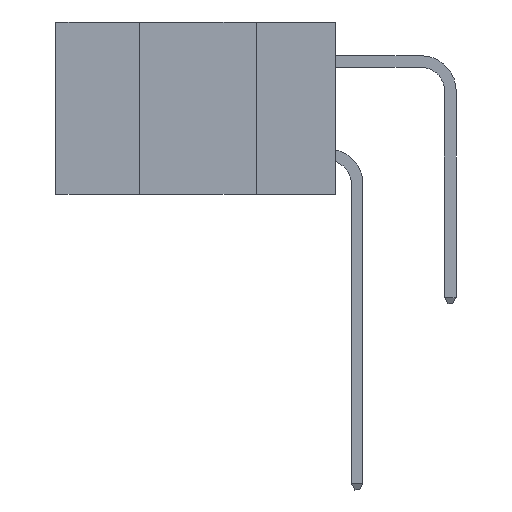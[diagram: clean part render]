
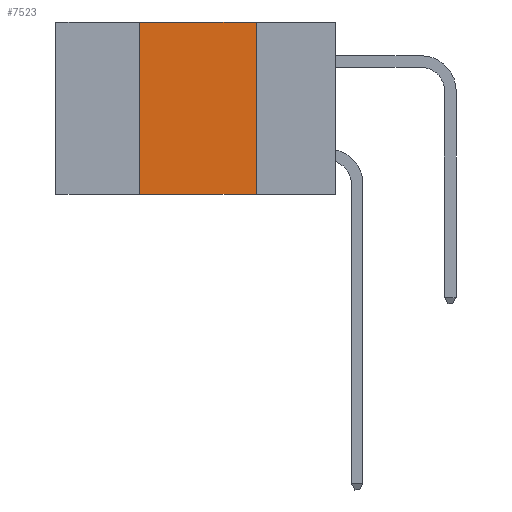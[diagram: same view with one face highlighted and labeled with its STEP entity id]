
A CAD part, left-side view. The second image highlights one B-rep face of the part: STEP entity #7523.
In plain terms, the highlighted planar face has unit normal (-1, 0, 0).
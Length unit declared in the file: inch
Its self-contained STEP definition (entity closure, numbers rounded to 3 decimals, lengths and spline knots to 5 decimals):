
#45 = VERTEX_POINT ( 'NONE', #9979 ) ;
#201 = EDGE_CURVE ( 'NONE', #1730, #12419, #2643, .T. ) ;
#700 = ORIENTED_EDGE ( 'NONE', *, *, #6116, .F. ) ;
#1730 = VERTEX_POINT ( 'NONE', #5915 ) ;
#2170 = CARTESIAN_POINT ( 'NONE',  ( 0., 0.42, -0.37 ) ) ;
#2408 = CARTESIAN_POINT ( 'NONE',  ( 0., 0.42, 0. ) ) ;
#2643 = LINE ( 'NONE', #6814, #6777 ) ;
#3211 = DIRECTION ( 'NONE',  ( 0., 0., -1. ) ) ;
#3374 = VECTOR ( 'NONE', #3211, 39.37008 ) ;
#4611 = LINE ( 'NONE', #2408, #6084 ) ;
#5298 = ORIENTED_EDGE ( 'NONE', *, *, #201, .F. ) ;
#5835 = LINE ( 'NONE', #9090, #9541 ) ;
#5915 = CARTESIAN_POINT ( 'NONE',  ( 0., 0.42, 0. ) ) ;
#5981 = EDGE_CURVE ( 'NONE', #12419, #45, #6967, .T. ) ;
#6084 = VECTOR ( 'NONE', #6334, 39.37008 ) ;
#6116 = EDGE_CURVE ( 'NONE', #7684, #1730, #4611, .T. ) ;
#6334 = DIRECTION ( 'NONE',  ( 0., 0., 1. ) ) ;
#6777 = VECTOR ( 'NONE', #9034, 39.37008 ) ;
#6814 = CARTESIAN_POINT ( 'NONE',  ( 0., 0.6, 0. ) ) ;
#6967 = LINE ( 'NONE', #9605, #3374 ) ;
#7170 = FACE_OUTER_BOUND ( 'NONE', #7310, .T. ) ;
#7310 = EDGE_LOOP ( 'NONE', ( #8000, #5298, #700, #11504 ) ) ;
#7523 = ADVANCED_FACE ( 'NONE', ( #7170 ), #13474, .F. ) ;
#7684 = VERTEX_POINT ( 'NONE', #2170 ) ;
#8000 = ORIENTED_EDGE ( 'NONE', *, *, #5981, .F. ) ;
#8024 = DIRECTION ( 'NONE',  ( 0., -1., 0. ) ) ;
#9034 = DIRECTION ( 'NONE',  ( 0., -1., 0. ) ) ;
#9090 = CARTESIAN_POINT ( 'NONE',  ( 0., 0.6, -0.37 ) ) ;
#9541 = VECTOR ( 'NONE', #8024, 39.37008 ) ;
#9605 = CARTESIAN_POINT ( 'NONE',  ( 0., 0.17, 0. ) ) ;
#9979 = CARTESIAN_POINT ( 'NONE',  ( 0., 0.17, -0.37 ) ) ;
#10216 = CARTESIAN_POINT ( 'NONE',  ( 0., 0.6, 0. ) ) ;
#10710 = AXIS2_PLACEMENT_3D ( 'NONE', #10216, #11241, #13624 ) ;
#11241 = DIRECTION ( 'NONE',  ( 1., 0., 0. ) ) ;
#11504 = ORIENTED_EDGE ( 'NONE', *, *, #13467, .T. ) ;
#12419 = VERTEX_POINT ( 'NONE', #14013 ) ;
#13467 = EDGE_CURVE ( 'NONE', #7684, #45, #5835, .T. ) ;
#13474 = PLANE ( 'NONE',  #10710 ) ;
#13624 = DIRECTION ( 'NONE',  ( 0., 0., -1. ) ) ;
#14013 = CARTESIAN_POINT ( 'NONE',  ( 0., 0.17, 0. ) ) ;
